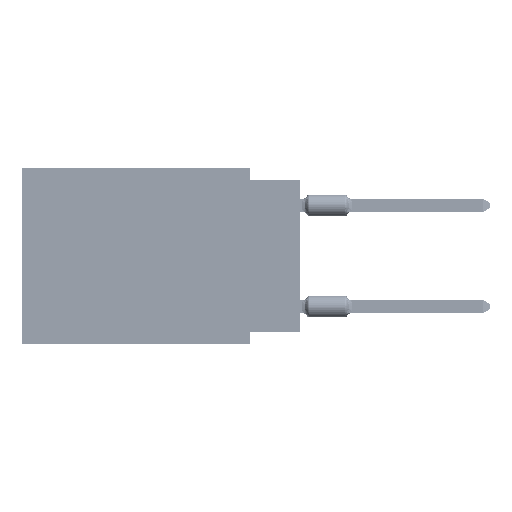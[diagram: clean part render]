
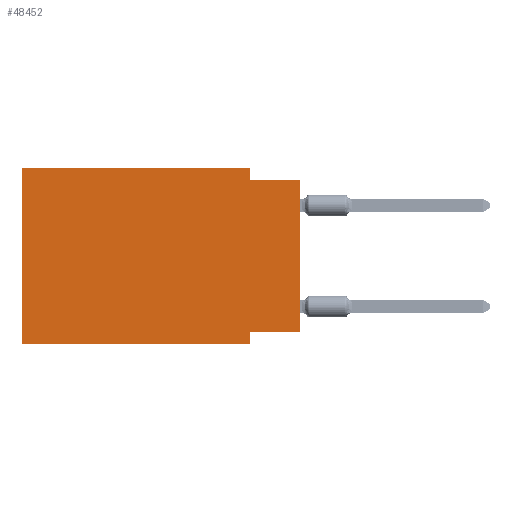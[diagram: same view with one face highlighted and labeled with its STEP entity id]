
A CAD part, left-side view. The second image highlights one B-rep face of the part: STEP entity #48452.
In plain terms, the highlighted planar face has unit normal (-1, 0, 0).
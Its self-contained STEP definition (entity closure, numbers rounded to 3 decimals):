
#200 = CARTESIAN_POINT ( 'NONE',  ( 0., 13.97, 0. ) ) ;
#1476 = ORIENTED_EDGE ( 'NONE', *, *, #6276, .F. ) ;
#1482 = LINE ( 'NONE', #22206, #37360 ) ;
#2534 = DIRECTION ( 'NONE',  ( 0., 0., 1. ) ) ;
#2957 = VECTOR ( 'NONE', #2534, 1000. ) ;
#4738 = VECTOR ( 'NONE', #30907, 1000. ) ;
#5311 = CARTESIAN_POINT ( 'NONE',  ( 0., 2.54, -8.255 ) ) ;
#5429 = DIRECTION ( 'NONE',  ( 1., 0., 0. ) ) ;
#6276 = EDGE_CURVE ( 'NONE', #10820, #7053, #22597, .T. ) ;
#6773 = ORIENTED_EDGE ( 'NONE', *, *, #38578, .F. ) ;
#7053 = VERTEX_POINT ( 'NONE', #5311 ) ;
#8300 = EDGE_CURVE ( 'NONE', #33714, #35138, #31132, .T. ) ;
#8959 = CARTESIAN_POINT ( 'NONE',  ( 0., 13.97, 0. ) ) ;
#10566 = LINE ( 'NONE', #30940, #24475 ) ;
#10570 = EDGE_LOOP ( 'NONE', ( #48072, #56664, #49328, #39875, #22011, #64596, #6773, #1476 ) ) ;
#10820 = VERTEX_POINT ( 'NONE', #51409 ) ;
#12089 = PLANE ( 'NONE',  #46871 ) ;
#13169 = LINE ( 'NONE', #63938, #35203 ) ;
#13537 = CARTESIAN_POINT ( 'NONE',  ( 0., 0., 0. ) ) ;
#16127 = EDGE_CURVE ( 'NONE', #24936, #38837, #10566, .T. ) ;
#17031 = CARTESIAN_POINT ( 'NONE',  ( 0., 13.97, -8.89 ) ) ;
#17763 = CARTESIAN_POINT ( 'NONE',  ( 0., 2.54, -8.89 ) ) ;
#19781 = DIRECTION ( 'NONE',  ( 0., -1., 0. ) ) ;
#21804 = DIRECTION ( 'NONE',  ( 0., 0., -1. ) ) ;
#21877 = DIRECTION ( 'NONE',  ( 0., 0., -1. ) ) ;
#22011 = ORIENTED_EDGE ( 'NONE', *, *, #38183, .F. ) ;
#22206 = CARTESIAN_POINT ( 'NONE',  ( 0., 2.54, 0. ) ) ;
#22597 = LINE ( 'NONE', #62340, #41755 ) ;
#24475 = VECTOR ( 'NONE', #45979, 1000. ) ;
#24936 = VERTEX_POINT ( 'NONE', #17031 ) ;
#25771 = EDGE_CURVE ( 'NONE', #40433, #38241, #52280, .T. ) ;
#26800 = FACE_OUTER_BOUND ( 'NONE', #10570, .T. ) ;
#30907 = DIRECTION ( 'NONE',  ( 0., -1., 0. ) ) ;
#30940 = CARTESIAN_POINT ( 'NONE',  ( 0., 13.97, -8.89 ) ) ;
#31132 = LINE ( 'NONE', #65544, #59534 ) ;
#33117 = VECTOR ( 'NONE', #21804, 1000. ) ;
#33272 = LINE ( 'NONE', #13537, #2957 ) ;
#33714 = VERTEX_POINT ( 'NONE', #50201 ) ;
#35138 = VERTEX_POINT ( 'NONE', #56213 ) ;
#35203 = VECTOR ( 'NONE', #52926, 1000. ) ;
#36155 = CARTESIAN_POINT ( 'NONE',  ( 0., 13.97, 0. ) ) ;
#37360 = VECTOR ( 'NONE', #21877, 1000. ) ;
#37925 = DIRECTION ( 'NONE',  ( 0., 1., 0. ) ) ;
#38183 = EDGE_CURVE ( 'NONE', #24936, #40433, #13169, .T. ) ;
#38209 = CARTESIAN_POINT ( 'NONE',  ( 0., 2.54, 0. ) ) ;
#38241 = VERTEX_POINT ( 'NONE', #38209 ) ;
#38578 = EDGE_CURVE ( 'NONE', #7053, #38837, #48495, .T. ) ;
#38837 = VERTEX_POINT ( 'NONE', #63859 ) ;
#39875 = ORIENTED_EDGE ( 'NONE', *, *, #25771, .F. ) ;
#40433 = VERTEX_POINT ( 'NONE', #8959 ) ;
#41755 = VECTOR ( 'NONE', #37925, 1000. ) ;
#45979 = DIRECTION ( 'NONE',  ( 0., -1., 0. ) ) ;
#46495 = EDGE_CURVE ( 'NONE', #10820, #35138, #33272, .T. ) ;
#46871 = AXIS2_PLACEMENT_3D ( 'NONE', #36155, #5429, #51524 ) ;
#48072 = ORIENTED_EDGE ( 'NONE', *, *, #46495, .T. ) ;
#48452 = ADVANCED_FACE ( 'NONE', ( #26800 ), #12089, .F. ) ;
#48495 = LINE ( 'NONE', #17763, #33117 ) ;
#49328 = ORIENTED_EDGE ( 'NONE', *, *, #59620, .F. ) ;
#50201 = CARTESIAN_POINT ( 'NONE',  ( 0., 2.54, -0.635 ) ) ;
#51409 = CARTESIAN_POINT ( 'NONE',  ( 0., 0., -8.255 ) ) ;
#51524 = DIRECTION ( 'NONE',  ( 0., 0., -1. ) ) ;
#52280 = LINE ( 'NONE', #200, #4738 ) ;
#52926 = DIRECTION ( 'NONE',  ( 0., 0., 1. ) ) ;
#56213 = CARTESIAN_POINT ( 'NONE',  ( 0., 0., -0.635 ) ) ;
#56664 = ORIENTED_EDGE ( 'NONE', *, *, #8300, .F. ) ;
#59534 = VECTOR ( 'NONE', #19781, 1000. ) ;
#59620 = EDGE_CURVE ( 'NONE', #38241, #33714, #1482, .T. ) ;
#62340 = CARTESIAN_POINT ( 'NONE',  ( 0., 0., -8.255 ) ) ;
#63859 = CARTESIAN_POINT ( 'NONE',  ( 0., 2.54, -8.89 ) ) ;
#63938 = CARTESIAN_POINT ( 'NONE',  ( 0., 13.97, 0. ) ) ;
#64596 = ORIENTED_EDGE ( 'NONE', *, *, #16127, .T. ) ;
#65544 = CARTESIAN_POINT ( 'NONE',  ( 0., 0., -0.635 ) ) ;
